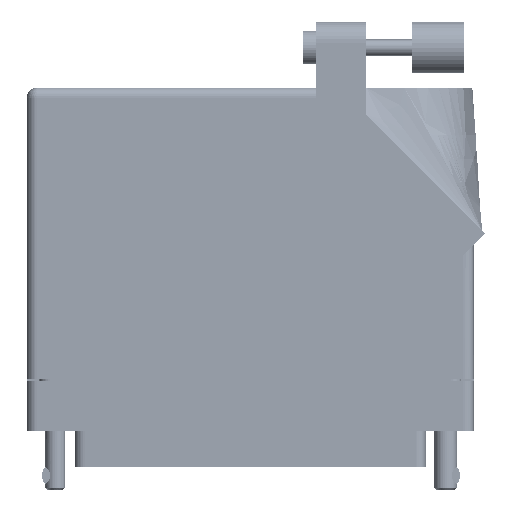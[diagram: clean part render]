
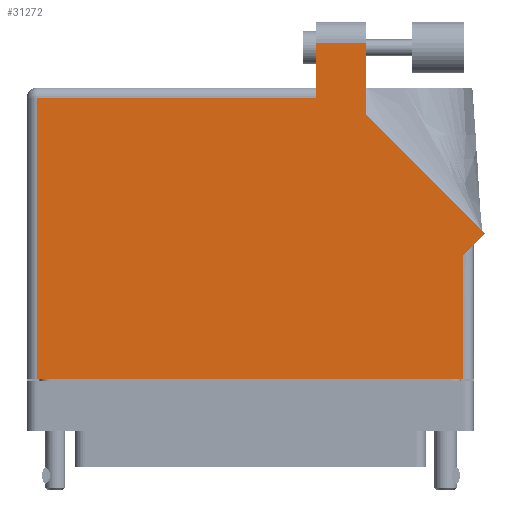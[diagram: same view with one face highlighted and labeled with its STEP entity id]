
A CAD part, front view. The second image highlights one B-rep face of the part: STEP entity #31272.
In plain terms, the highlighted face is planar.
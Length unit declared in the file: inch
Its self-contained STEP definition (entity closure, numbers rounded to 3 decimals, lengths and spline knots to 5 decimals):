
#368 = CARTESIAN_POINT ( 'NONE',  ( -1.297, -0.1, 0.617 ) ) ;
#3453 = VECTOR ( 'NONE', #23239, 39.37008 ) ;
#4998 = DIRECTION ( 'NONE',  ( -1., 0., 0. ) ) ;
#5408 = CARTESIAN_POINT ( 'NONE',  ( 0.399, 1.95, 0.617 ) ) ;
#7288 = LINE ( 'NONE', #51448, #16524 ) ;
#7494 = LINE ( 'NONE', #24764, #53192 ) ;
#8870 = EDGE_CURVE ( 'NONE', #30177, #51873, #83068, .T. ) ;
#10704 = VECTOR ( 'NONE', #56953, 39.37008 ) ;
#10855 = LINE ( 'NONE', #70941, #13926 ) ;
#13392 = LINE ( 'NONE', #16999, #40868 ) ;
#13926 = VECTOR ( 'NONE', #32324, 39.37008 ) ;
#14008 = FACE_OUTER_BOUND ( 'NONE', #75205, .T. ) ;
#16065 = CARTESIAN_POINT ( 'NONE',  ( 0.706, 1.95, 0.617 ) ) ;
#16524 = VECTOR ( 'NONE', #26193, 39.37008 ) ;
#16837 = LINE ( 'NONE', #23768, #10704 ) ;
#16999 = CARTESIAN_POINT ( 'NONE',  ( -1.359, 1.613, 0.617 ) ) ;
#20491 = VERTEX_POINT ( 'NONE', #59156 ) ;
#21242 = LINE ( 'NONE', #5408, #48682 ) ;
#23239 = DIRECTION ( 'NONE',  ( 0., 1., 0. ) ) ;
#23768 = CARTESIAN_POINT ( 'NONE',  ( -1.297, -0.1, 0.617 ) ) ;
#24587 = VERTEX_POINT ( 'NONE', #16065 ) ;
#24764 = CARTESIAN_POINT ( 'NONE',  ( 1.359, 0.715, 0.617 ) ) ;
#26026 = CARTESIAN_POINT ( 'NONE',  ( 1.42971, 0.78571, 0.617 ) ) ;
#26193 = DIRECTION ( 'NONE',  ( 0., 1., 0. ) ) ;
#28431 = VERTEX_POINT ( 'NONE', #26026 ) ;
#30177 = VERTEX_POINT ( 'NONE', #78582 ) ;
#31272 = ADVANCED_FACE ( 'NONE', ( #14008 ), #61330, .F. ) ;
#32084 = CARTESIAN_POINT ( 'NONE',  ( 0.706, 1.50942, 0.617 ) ) ;
#32147 = CARTESIAN_POINT ( 'NONE',  ( 0.399, 1.675, 0.617 ) ) ;
#32324 = DIRECTION ( 'NONE',  ( -0.707, 0.707, 0. ) ) ;
#32948 = LINE ( 'NONE', #62078, #3453 ) ;
#33022 = CARTESIAN_POINT ( 'NONE',  ( 0.399, 1.613, 0.617 ) ) ;
#35609 = CARTESIAN_POINT ( 'NONE',  ( -1.359, -0.1, 0.617 ) ) ;
#36472 = EDGE_CURVE ( 'NONE', #24587, #30177, #21242, .T. ) ;
#39435 = VERTEX_POINT ( 'NONE', #368 ) ;
#40160 = DIRECTION ( 'NONE',  ( 0., 0., -1. ) ) ;
#40868 = VECTOR ( 'NONE', #4998, 39.37008 ) ;
#42339 = EDGE_CURVE ( 'NONE', #28431, #75515, #10855, .T. ) ;
#42755 = ORIENTED_EDGE ( 'NONE', *, *, #73732, .T. ) ;
#42912 = EDGE_CURVE ( 'NONE', #39435, #55466, #83607, .T. ) ;
#43427 = ORIENTED_EDGE ( 'NONE', *, *, #42912, .T. ) ;
#44636 = EDGE_CURVE ( 'NONE', #75515, #24587, #7288, .T. ) ;
#44859 = DIRECTION ( 'NONE',  ( -1., 0., 0. ) ) ;
#45103 = ORIENTED_EDGE ( 'NONE', *, *, #36472, .T. ) ;
#46828 = DIRECTION ( 'NONE',  ( -1., 0., 0. ) ) ;
#47171 = AXIS2_PLACEMENT_3D ( 'NONE', #75457, #40160, #46828 ) ;
#48682 = VECTOR ( 'NONE', #44859, 39.37008 ) ;
#49519 = EDGE_CURVE ( 'NONE', #55466, #20491, #32948, .T. ) ;
#50293 = DIRECTION ( 'NONE',  ( 0.707, 0.707, 0. ) ) ;
#50793 = ORIENTED_EDGE ( 'NONE', *, *, #61082, .T. ) ;
#51448 = CARTESIAN_POINT ( 'NONE',  ( 0.706, 1.50942, 0.617 ) ) ;
#51736 = DIRECTION ( 'NONE',  ( 0., -1., 0. ) ) ;
#51873 = VERTEX_POINT ( 'NONE', #33022 ) ;
#53192 = VECTOR ( 'NONE', #50293, 39.37008 ) ;
#54921 = DIRECTION ( 'NONE',  ( 1., 0., 0. ) ) ;
#55466 = VERTEX_POINT ( 'NONE', #56971 ) ;
#56953 = DIRECTION ( 'NONE',  ( 0., -1., 0. ) ) ;
#56971 = CARTESIAN_POINT ( 'NONE',  ( 1.297, -0.1, 0.617 ) ) ;
#58378 = ORIENTED_EDGE ( 'NONE', *, *, #74646, .T. ) ;
#59156 = CARTESIAN_POINT ( 'NONE',  ( 1.297, 0.653, 0.617 ) ) ;
#60527 = ORIENTED_EDGE ( 'NONE', *, *, #42339, .T. ) ;
#61082 = EDGE_CURVE ( 'NONE', #83312, #39435, #16837, .T. ) ;
#61330 = PLANE ( 'NONE',  #47171 ) ;
#62010 = CARTESIAN_POINT ( 'NONE',  ( -1.297, 1.613, 0.617 ) ) ;
#62078 = CARTESIAN_POINT ( 'NONE',  ( 1.297, 0.715, 0.617 ) ) ;
#62717 = ORIENTED_EDGE ( 'NONE', *, *, #8870, .T. ) ;
#70941 = CARTESIAN_POINT ( 'NONE',  ( 1.42971, 0.78571, 0.617 ) ) ;
#71917 = VECTOR ( 'NONE', #51736, 39.37008 ) ;
#73732 = EDGE_CURVE ( 'NONE', #20491, #28431, #7494, .T. ) ;
#74646 = EDGE_CURVE ( 'NONE', #51873, #83312, #13392, .T. ) ;
#75205 = EDGE_LOOP ( 'NONE', ( #77880, #45103, #62717, #58378, #50793, #43427, #83087, #42755, #60527 ) ) ;
#75457 = CARTESIAN_POINT ( 'NONE',  ( -1.359, 1.675, 0.617 ) ) ;
#75515 = VERTEX_POINT ( 'NONE', #32084 ) ;
#77880 = ORIENTED_EDGE ( 'NONE', *, *, #44636, .T. ) ;
#78582 = CARTESIAN_POINT ( 'NONE',  ( 0.399, 1.95, 0.617 ) ) ;
#78615 = VECTOR ( 'NONE', #54921, 39.37008 ) ;
#83068 = LINE ( 'NONE', #32147, #71917 ) ;
#83087 = ORIENTED_EDGE ( 'NONE', *, *, #49519, .T. ) ;
#83312 = VERTEX_POINT ( 'NONE', #62010 ) ;
#83607 = LINE ( 'NONE', #35609, #78615 ) ;
